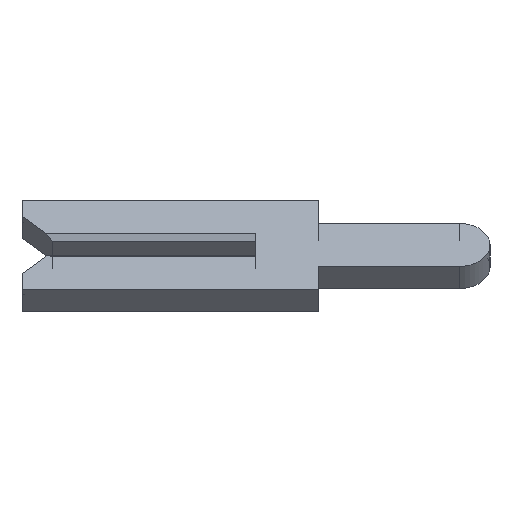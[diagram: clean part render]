
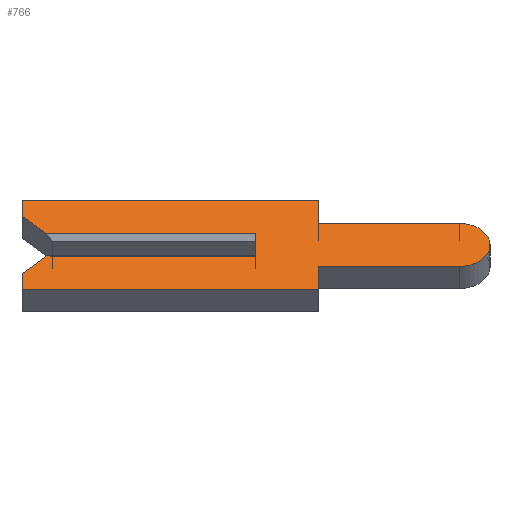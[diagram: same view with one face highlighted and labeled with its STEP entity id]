
A CAD part, left-side view. The second image highlights one B-rep face of the part: STEP entity #766.
In plain terms, the highlighted face is planar.
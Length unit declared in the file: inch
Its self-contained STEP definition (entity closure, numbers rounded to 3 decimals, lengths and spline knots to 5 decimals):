
#1 = CARTESIAN_POINT ( 'NONE',  ( -0.01, -0.04, -0.0195 ) ) ;
#26 = VECTOR ( 'NONE', #2502, 39.37008 ) ;
#79 = VERTEX_POINT ( 'NONE', #2418 ) ;
#105 = CARTESIAN_POINT ( 'NONE',  ( -0.01, -0.04, -0.0195 ) ) ;
#106 = DIRECTION ( 'NONE',  ( 0., 0., 1. ) ) ;
#121 = DIRECTION ( 'NONE',  ( 0., -0.707, 0.707 ) ) ;
#132 = VERTEX_POINT ( 'NONE', #978 ) ;
#154 = AXIS2_PLACEMENT_3D ( 'NONE', #1448, #2082, #283 ) ;
#189 = CARTESIAN_POINT ( 'NONE',  ( -0.01, 0.15, -0.04 ) ) ;
#244 = VECTOR ( 'NONE', #1469, 39.37008 ) ;
#257 = EDGE_CURVE ( 'NONE', #132, #2325, #609, .T. ) ;
#283 = DIRECTION ( 'NONE',  ( 0., 0., -1. ) ) ;
#286 = EDGE_LOOP ( 'NONE', ( #2241, #2445, #2313, #1936, #311, #2002, #1497, #584, #1083, #1228, #2083, #1890, #1153, #2188 ) ) ;
#311 = ORIENTED_EDGE ( 'NONE', *, *, #917, .F. ) ;
#356 = CARTESIAN_POINT ( 'NONE',  ( -0.01, 0.15, 0.026 ) ) ;
#387 = EDGE_CURVE ( 'NONE', #2054, #1283, #1843, .T. ) ;
#391 = CARTESIAN_POINT ( 'NONE',  ( -0.01, -0.1305, 0.0195 ) ) ;
#397 = CARTESIAN_POINT ( 'NONE',  ( -0.01, 0., 0.0065 ) ) ;
#423 = VECTOR ( 'NONE', #2222, 39.37008 ) ;
#453 = DIRECTION ( 'NONE',  ( 0., 0., -1. ) ) ;
#459 = CARTESIAN_POINT ( 'NONE',  ( -0.01, -0.1305, -0.01 ) ) ;
#492 = EDGE_CURVE ( 'NONE', #2159, #1859, #1468, .T. ) ;
#501 = CARTESIAN_POINT ( 'NONE',  ( -0.01, 0.15, 0.04 ) ) ;
#560 = CARTESIAN_POINT ( 'NONE',  ( -0.01, -0.1305, -0.0195 ) ) ;
#576 = CARTESIAN_POINT ( 'NONE',  ( -0.01, 0.134, 0.01 ) ) ;
#584 = ORIENTED_EDGE ( 'NONE', *, *, #2231, .F. ) ;
#587 = DIRECTION ( 'NONE',  ( 0., 0., 1. ) ) ;
#609 = LINE ( 'NONE', #1438, #1425 ) ;
#613 = DIRECTION ( 'NONE',  ( 0., 1., 0. ) ) ;
#617 = EDGE_CURVE ( 'NONE', #1894, #79, #1455, .T. ) ;
#686 = EDGE_CURVE ( 'NONE', #2256, #2159, #1265, .T. ) ;
#701 = CARTESIAN_POINT ( 'NONE',  ( -0.01, 0.15, -0.026 ) ) ;
#733 = VECTOR ( 'NONE', #121, 39.37008 ) ;
#761 = CARTESIAN_POINT ( 'NONE',  ( -0.01, 0.134, -0.01 ) ) ;
#766 = ADVANCED_FACE ( 'NONE', ( #1338 ), #842, .F. ) ;
#791 = LINE ( 'NONE', #1058, #1651 ) ;
#795 = CARTESIAN_POINT ( 'NONE',  ( -0.01, -0.04, 0.0195 ) ) ;
#825 = LINE ( 'NONE', #1505, #1844 ) ;
#842 = PLANE ( 'NONE',  #2468 ) ;
#851 = VECTOR ( 'NONE', #1653, 39.37008 ) ;
#917 = EDGE_CURVE ( 'NONE', #2325, #1241, #791, .T. ) ;
#978 = CARTESIAN_POINT ( 'NONE',  ( -0.01, -0.04, -0.04 ) ) ;
#1007 = LINE ( 'NONE', #2019, #423 ) ;
#1058 = CARTESIAN_POINT ( 'NONE',  ( -0.01, 0.15, -0.026 ) ) ;
#1063 = EDGE_CURVE ( 'NONE', #2118, #132, #2552, .T. ) ;
#1070 = CARTESIAN_POINT ( 'NONE',  ( -0.01, 0.1305, 0.0065 ) ) ;
#1072 = LINE ( 'NONE', #105, #2518 ) ;
#1083 = ORIENTED_EDGE ( 'NONE', *, *, #492, .F. ) ;
#1085 = DIRECTION ( 'NONE',  ( 0., 0., -1. ) ) ;
#1102 = EDGE_CURVE ( 'NONE', #2290, #1125, #2423, .T. ) ;
#1107 = CARTESIAN_POINT ( 'NONE',  ( -0.01, 0., 0.01 ) ) ;
#1124 = DIRECTION ( 'NONE',  ( 0., 0., 1. ) ) ;
#1125 = VERTEX_POINT ( 'NONE', #2544 ) ;
#1153 = ORIENTED_EDGE ( 'NONE', *, *, #1794, .F. ) ;
#1170 = LINE ( 'NONE', #356, #2070 ) ;
#1228 = ORIENTED_EDGE ( 'NONE', *, *, #686, .F. ) ;
#1241 = VERTEX_POINT ( 'NONE', #701 ) ;
#1265 = LINE ( 'NONE', #2309, #851 ) ;
#1283 = VERTEX_POINT ( 'NONE', #1697 ) ;
#1302 = CARTESIAN_POINT ( 'NONE',  ( -0.01, 0.1305, -0.0065 ) ) ;
#1338 = FACE_OUTER_BOUND ( 'NONE', #286, .T. ) ;
#1375 = EDGE_CURVE ( 'NONE', #1125, #2256, #825, .T. ) ;
#1423 = DIRECTION ( 'NONE',  ( 0., 1., 0. ) ) ;
#1425 = VECTOR ( 'NONE', #1423, 39.37008 ) ;
#1427 = LINE ( 'NONE', #397, #1717 ) ;
#1438 = CARTESIAN_POINT ( 'NONE',  ( -0.01, 0.15, -0.04 ) ) ;
#1448 = CARTESIAN_POINT ( 'NONE',  ( -0.01, -0.1305, 0. ) ) ;
#1455 = LINE ( 'NONE', #459, #244 ) ;
#1463 = CARTESIAN_POINT ( 'NONE',  ( -0.01, -0.1305, 0. ) ) ;
#1468 = CIRCLE ( 'NONE', #154, 0.0195 ) ;
#1469 = DIRECTION ( 'NONE',  ( 0., -1., 0. ) ) ;
#1473 = EDGE_CURVE ( 'NONE', #1241, #1894, #1982, .T. ) ;
#1490 = DIRECTION ( 'NONE',  ( 0., -1., 0. ) ) ;
#1497 = ORIENTED_EDGE ( 'NONE', *, *, #1063, .F. ) ;
#1505 = CARTESIAN_POINT ( 'NONE',  ( -0.01, -0.04, 0.04 ) ) ;
#1604 = VERTEX_POINT ( 'NONE', #1107 ) ;
#1614 = CARTESIAN_POINT ( 'NONE',  ( -0.01, 0.15, 0.04 ) ) ;
#1651 = VECTOR ( 'NONE', #106, 39.37008 ) ;
#1653 = DIRECTION ( 'NONE',  ( 0., -1., 0. ) ) ;
#1659 = DIRECTION ( 'NONE',  ( 1., 0., 0. ) ) ;
#1697 = CARTESIAN_POINT ( 'NONE',  ( -0.01, 0.15, 0.026 ) ) ;
#1709 = CARTESIAN_POINT ( 'NONE',  ( -0.01, -0.04, -0.04 ) ) ;
#1717 = VECTOR ( 'NONE', #587, 39.37008 ) ;
#1794 = EDGE_CURVE ( 'NONE', #1283, #2290, #1170, .T. ) ;
#1843 = LINE ( 'NONE', #1070, #26 ) ;
#1844 = VECTOR ( 'NONE', #1085, 39.37008 ) ;
#1859 = VERTEX_POINT ( 'NONE', #560 ) ;
#1880 = VECTOR ( 'NONE', #1490, 39.37008 ) ;
#1890 = ORIENTED_EDGE ( 'NONE', *, *, #1102, .F. ) ;
#1894 = VERTEX_POINT ( 'NONE', #761 ) ;
#1936 = ORIENTED_EDGE ( 'NONE', *, *, #1473, .F. ) ;
#1982 = LINE ( 'NONE', #1302, #733 ) ;
#2002 = ORIENTED_EDGE ( 'NONE', *, *, #257, .F. ) ;
#2019 = CARTESIAN_POINT ( 'NONE',  ( -0.01, 0.15, 0.01 ) ) ;
#2054 = VERTEX_POINT ( 'NONE', #576 ) ;
#2070 = VECTOR ( 'NONE', #1124, 39.37008 ) ;
#2082 = DIRECTION ( 'NONE',  ( 1., 0., 0. ) ) ;
#2083 = ORIENTED_EDGE ( 'NONE', *, *, #1375, .F. ) ;
#2118 = VERTEX_POINT ( 'NONE', #1 ) ;
#2159 = VERTEX_POINT ( 'NONE', #391 ) ;
#2188 = ORIENTED_EDGE ( 'NONE', *, *, #387, .F. ) ;
#2222 = DIRECTION ( 'NONE',  ( 0., -1., 0. ) ) ;
#2231 = EDGE_CURVE ( 'NONE', #1859, #2118, #1072, .T. ) ;
#2241 = ORIENTED_EDGE ( 'NONE', *, *, #2427, .T. ) ;
#2256 = VERTEX_POINT ( 'NONE', #795 ) ;
#2290 = VERTEX_POINT ( 'NONE', #1614 ) ;
#2309 = CARTESIAN_POINT ( 'NONE',  ( -0.01, -0.04, 0.0195 ) ) ;
#2313 = ORIENTED_EDGE ( 'NONE', *, *, #617, .F. ) ;
#2325 = VERTEX_POINT ( 'NONE', #189 ) ;
#2342 = EDGE_CURVE ( 'NONE', #79, #1604, #1427, .T. ) ;
#2418 = CARTESIAN_POINT ( 'NONE',  ( -0.01, 0., -0.01 ) ) ;
#2423 = LINE ( 'NONE', #501, #1880 ) ;
#2427 = EDGE_CURVE ( 'NONE', #2054, #1604, #1007, .T. ) ;
#2445 = ORIENTED_EDGE ( 'NONE', *, *, #2342, .F. ) ;
#2457 = VECTOR ( 'NONE', #2526, 39.37008 ) ;
#2468 = AXIS2_PLACEMENT_3D ( 'NONE', #1463, #1659, #453 ) ;
#2502 = DIRECTION ( 'NONE',  ( 0., 0.707, 0.707 ) ) ;
#2518 = VECTOR ( 'NONE', #613, 39.37008 ) ;
#2526 = DIRECTION ( 'NONE',  ( 0., 0., -1. ) ) ;
#2544 = CARTESIAN_POINT ( 'NONE',  ( -0.01, -0.04, 0.04 ) ) ;
#2552 = LINE ( 'NONE', #1709, #2457 ) ;
